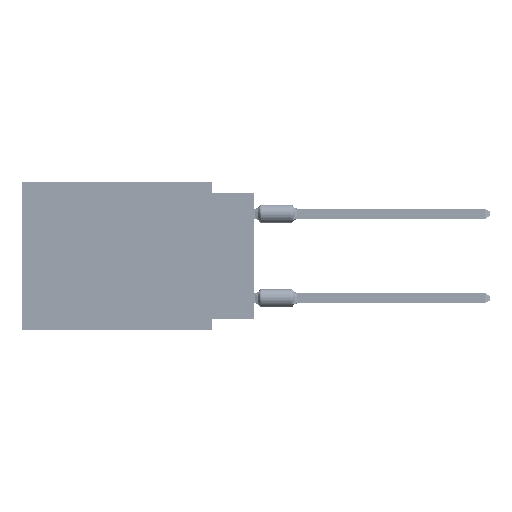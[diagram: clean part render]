
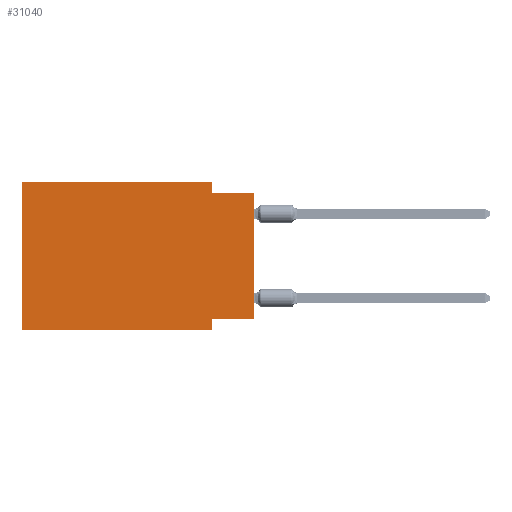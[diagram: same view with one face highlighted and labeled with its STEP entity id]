
A CAD part, left-side view. The second image highlights one B-rep face of the part: STEP entity #31040.
In plain terms, the highlighted planar face has unit normal (-1, 0, 0).
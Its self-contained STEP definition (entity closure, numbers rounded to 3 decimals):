
#3208 = VECTOR ( 'NONE', #78188, 1000. ) ;
#4026 = CARTESIAN_POINT ( 'NONE',  ( 0., 13.97, -8.89 ) ) ;
#4341 = EDGE_CURVE ( 'NONE', #16478, #9707, #44254, .T. ) ;
#4693 = VECTOR ( 'NONE', #70107, 1000. ) ;
#5955 = CARTESIAN_POINT ( 'NONE',  ( 0., 2.54, 0. ) ) ;
#6572 = ORIENTED_EDGE ( 'NONE', *, *, #44943, .F. ) ;
#7831 = EDGE_CURVE ( 'NONE', #40860, #48059, #72261, .T. ) ;
#9707 = VERTEX_POINT ( 'NONE', #41808 ) ;
#11878 = EDGE_LOOP ( 'NONE', ( #57796, #21111, #57170, #41715, #66856, #51459, #26230, #6572 ) ) ;
#13532 = EDGE_CURVE ( 'NONE', #58798, #16632, #34535, .T. ) ;
#15875 = VERTEX_POINT ( 'NONE', #32315 ) ;
#15896 = LINE ( 'NONE', #40087, #58109 ) ;
#16190 = LINE ( 'NONE', #57852, #29416 ) ;
#16366 = AXIS2_PLACEMENT_3D ( 'NONE', #24205, #17465, #77370 ) ;
#16478 = VERTEX_POINT ( 'NONE', #4026 ) ;
#16632 = VERTEX_POINT ( 'NONE', #53453 ) ;
#17465 = DIRECTION ( 'NONE',  ( 1., 0., 0. ) ) ;
#18251 = PLANE ( 'NONE',  #16366 ) ;
#21111 = ORIENTED_EDGE ( 'NONE', *, *, #40410, .F. ) ;
#24205 = CARTESIAN_POINT ( 'NONE',  ( 0., 13.97, 0. ) ) ;
#25067 = CARTESIAN_POINT ( 'NONE',  ( 0., 0., -8.255 ) ) ;
#25254 = DIRECTION ( 'NONE',  ( 0., 1., 0. ) ) ;
#25856 = CARTESIAN_POINT ( 'NONE',  ( 0., 2.54, -8.89 ) ) ;
#26124 = DIRECTION ( 'NONE',  ( 0., -1., 0. ) ) ;
#26230 = ORIENTED_EDGE ( 'NONE', *, *, #42225, .F. ) ;
#29122 = VECTOR ( 'NONE', #25254, 1000. ) ;
#29416 = VECTOR ( 'NONE', #63791, 1000. ) ;
#30132 = VECTOR ( 'NONE', #77380, 1000. ) ;
#30785 = CARTESIAN_POINT ( 'NONE',  ( 0., 13.97, 0. ) ) ;
#30882 = VERTEX_POINT ( 'NONE', #25856 ) ;
#31040 = ADVANCED_FACE ( 'NONE', ( #59116 ), #18251, .F. ) ;
#32315 = CARTESIAN_POINT ( 'NONE',  ( 0., 2.54, -8.255 ) ) ;
#33818 = EDGE_CURVE ( 'NONE', #16478, #30882, #16190, .T. ) ;
#34535 = LINE ( 'NONE', #5955, #30132 ) ;
#37530 = LINE ( 'NONE', #55377, #29122 ) ;
#38484 = VECTOR ( 'NONE', #26124, 1000. ) ;
#40087 = CARTESIAN_POINT ( 'NONE',  ( 0., 2.54, -8.89 ) ) ;
#40410 = EDGE_CURVE ( 'NONE', #16632, #48059, #52249, .T. ) ;
#40860 = VERTEX_POINT ( 'NONE', #25067 ) ;
#41715 = ORIENTED_EDGE ( 'NONE', *, *, #67486, .F. ) ;
#41808 = CARTESIAN_POINT ( 'NONE',  ( 0., 13.97, 0. ) ) ;
#42225 = EDGE_CURVE ( 'NONE', #15875, #30882, #15896, .T. ) ;
#44254 = LINE ( 'NONE', #30785, #47161 ) ;
#44943 = EDGE_CURVE ( 'NONE', #40860, #15875, #37530, .T. ) ;
#45137 = CARTESIAN_POINT ( 'NONE',  ( 0., 13.97, 0. ) ) ;
#47161 = VECTOR ( 'NONE', #49804, 1000. ) ;
#48059 = VERTEX_POINT ( 'NONE', #52476 ) ;
#49804 = DIRECTION ( 'NONE',  ( 0., 0., 1. ) ) ;
#51459 = ORIENTED_EDGE ( 'NONE', *, *, #33818, .T. ) ;
#52249 = LINE ( 'NONE', #76834, #4693 ) ;
#52476 = CARTESIAN_POINT ( 'NONE',  ( 0., 0., -0.635 ) ) ;
#53453 = CARTESIAN_POINT ( 'NONE',  ( 0., 2.54, -0.635 ) ) ;
#55377 = CARTESIAN_POINT ( 'NONE',  ( 0., 0., -8.255 ) ) ;
#57170 = ORIENTED_EDGE ( 'NONE', *, *, #13532, .F. ) ;
#57796 = ORIENTED_EDGE ( 'NONE', *, *, #7831, .T. ) ;
#57852 = CARTESIAN_POINT ( 'NONE',  ( 0., 13.97, -8.89 ) ) ;
#58109 = VECTOR ( 'NONE', #64266, 1000. ) ;
#58798 = VERTEX_POINT ( 'NONE', #70293 ) ;
#59116 = FACE_OUTER_BOUND ( 'NONE', #11878, .T. ) ;
#63791 = DIRECTION ( 'NONE',  ( 0., -1., 0. ) ) ;
#64266 = DIRECTION ( 'NONE',  ( 0., 0., -1. ) ) ;
#66856 = ORIENTED_EDGE ( 'NONE', *, *, #4341, .F. ) ;
#67486 = EDGE_CURVE ( 'NONE', #9707, #58798, #68953, .T. ) ;
#68953 = LINE ( 'NONE', #45137, #38484 ) ;
#70107 = DIRECTION ( 'NONE',  ( 0., -1., 0. ) ) ;
#70293 = CARTESIAN_POINT ( 'NONE',  ( 0., 2.54, 0. ) ) ;
#72261 = LINE ( 'NONE', #76630, #3208 ) ;
#76630 = CARTESIAN_POINT ( 'NONE',  ( 0., 0., 0. ) ) ;
#76834 = CARTESIAN_POINT ( 'NONE',  ( 0., 0., -0.635 ) ) ;
#77370 = DIRECTION ( 'NONE',  ( 0., 0., -1. ) ) ;
#77380 = DIRECTION ( 'NONE',  ( 0., 0., -1. ) ) ;
#78188 = DIRECTION ( 'NONE',  ( 0., 0., 1. ) ) ;
